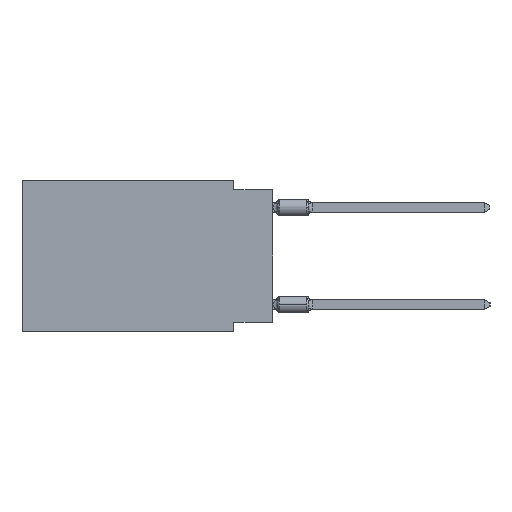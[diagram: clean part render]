
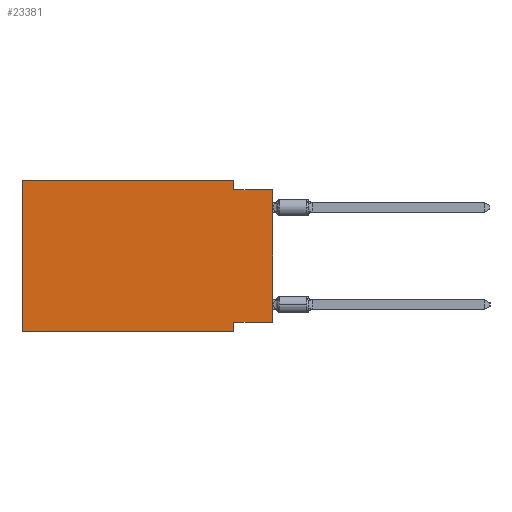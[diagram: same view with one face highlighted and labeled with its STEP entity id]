
A CAD part, left-side view. The second image highlights one B-rep face of the part: STEP entity #23381.
In plain terms, the highlighted planar face has unit normal (-1, 0, 0).
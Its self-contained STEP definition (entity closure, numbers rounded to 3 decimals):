
#74 = LINE ( 'NONE', #25284, #29090 ) ;
#258 = DIRECTION ( 'NONE',  ( 0., 0., 1. ) ) ;
#794 = DIRECTION ( 'NONE',  ( 0., 1., 0. ) ) ;
#1066 = VERTEX_POINT ( 'NONE', #29072 ) ;
#2124 = DIRECTION ( 'NONE',  ( 0., -1., 0. ) ) ;
#2370 = EDGE_CURVE ( 'NONE', #1066, #18489, #74, .T. ) ;
#3048 = LINE ( 'NONE', #8605, #16916 ) ;
#3217 = CARTESIAN_POINT ( 'NONE',  ( 0., 2.54, -0.635 ) ) ;
#3464 = EDGE_CURVE ( 'NONE', #25221, #15336, #23334, .T. ) ;
#4582 = ORIENTED_EDGE ( 'NONE', *, *, #31115, .F. ) ;
#4725 = DIRECTION ( 'NONE',  ( 0., -1., 0. ) ) ;
#5016 = DIRECTION ( 'NONE',  ( 0., 0., -1. ) ) ;
#5195 = DIRECTION ( 'NONE',  ( 1., 0., 0. ) ) ;
#6644 = VECTOR ( 'NONE', #794, 1000. ) ;
#6961 = VECTOR ( 'NONE', #2124, 1000. ) ;
#7699 = PLANE ( 'NONE',  #22214 ) ;
#8605 = CARTESIAN_POINT ( 'NONE',  ( 0., 16.383, 0. ) ) ;
#9693 = LINE ( 'NONE', #28014, #6644 ) ;
#10263 = EDGE_CURVE ( 'NONE', #18567, #1066, #9693, .T. ) ;
#10994 = CARTESIAN_POINT ( 'NONE',  ( 0., 16.383, 0. ) ) ;
#12427 = CARTESIAN_POINT ( 'NONE',  ( 0., 16.383, 0. ) ) ;
#13568 = LINE ( 'NONE', #24493, #6961 ) ;
#13570 = CARTESIAN_POINT ( 'NONE',  ( 0., 0., -0.635 ) ) ;
#14565 = VECTOR ( 'NONE', #5016, 1000. ) ;
#14622 = ORIENTED_EDGE ( 'NONE', *, *, #10263, .F. ) ;
#14913 = DIRECTION ( 'NONE',  ( 0., 0., 1. ) ) ;
#14944 = CARTESIAN_POINT ( 'NONE',  ( 0., 2.54, -9.906 ) ) ;
#14964 = VECTOR ( 'NONE', #4725, 1000. ) ;
#15336 = VERTEX_POINT ( 'NONE', #10994 ) ;
#16800 = DIRECTION ( 'NONE',  ( 0., -1., 0. ) ) ;
#16916 = VECTOR ( 'NONE', #16800, 1000. ) ;
#16941 = CARTESIAN_POINT ( 'NONE',  ( 0., 16.383, -9.906 ) ) ;
#17483 = LINE ( 'NONE', #28431, #14964 ) ;
#17745 = ORIENTED_EDGE ( 'NONE', *, *, #32402, .F. ) ;
#18145 = ORIENTED_EDGE ( 'NONE', *, *, #30326, .T. ) ;
#18489 = VERTEX_POINT ( 'NONE', #14944 ) ;
#18567 = VERTEX_POINT ( 'NONE', #28911 ) ;
#21264 = VERTEX_POINT ( 'NONE', #13570 ) ;
#21716 = ORIENTED_EDGE ( 'NONE', *, *, #25077, .T. ) ;
#22214 = AXIS2_PLACEMENT_3D ( 'NONE', #29540, #5195, #27568 ) ;
#23334 = LINE ( 'NONE', #12427, #29685 ) ;
#23381 = ADVANCED_FACE ( 'NONE', ( #31868 ), #7699, .F. ) ;
#24274 = VECTOR ( 'NONE', #258, 1000. ) ;
#24493 = CARTESIAN_POINT ( 'NONE',  ( 0., 16.383, -9.906 ) ) ;
#24734 = VERTEX_POINT ( 'NONE', #28099 ) ;
#24772 = CARTESIAN_POINT ( 'NONE',  ( 0., 0., 0. ) ) ;
#25077 = EDGE_CURVE ( 'NONE', #25221, #18489, #13568, .T. ) ;
#25221 = VERTEX_POINT ( 'NONE', #16941 ) ;
#25284 = CARTESIAN_POINT ( 'NONE',  ( 0., 2.54, -9.906 ) ) ;
#26261 = ORIENTED_EDGE ( 'NONE', *, *, #3464, .F. ) ;
#26264 = VERTEX_POINT ( 'NONE', #3217 ) ;
#26872 = EDGE_CURVE ( 'NONE', #26264, #21264, #17483, .T. ) ;
#27568 = DIRECTION ( 'NONE',  ( 0., 0., -1. ) ) ;
#27635 = DIRECTION ( 'NONE',  ( 0., 0., -1. ) ) ;
#28014 = CARTESIAN_POINT ( 'NONE',  ( 0., 0., -9.271 ) ) ;
#28099 = CARTESIAN_POINT ( 'NONE',  ( 0., 2.54, 0. ) ) ;
#28231 = ORIENTED_EDGE ( 'NONE', *, *, #2370, .F. ) ;
#28431 = CARTESIAN_POINT ( 'NONE',  ( 0., 0., -0.635 ) ) ;
#28911 = CARTESIAN_POINT ( 'NONE',  ( 0., 0., -9.271 ) ) ;
#29072 = CARTESIAN_POINT ( 'NONE',  ( 0., 2.54, -9.271 ) ) ;
#29090 = VECTOR ( 'NONE', #27635, 1000. ) ;
#29540 = CARTESIAN_POINT ( 'NONE',  ( 0., 16.383, 0. ) ) ;
#29685 = VECTOR ( 'NONE', #14913, 1000. ) ;
#30326 = EDGE_CURVE ( 'NONE', #18567, #21264, #32838, .T. ) ;
#31115 = EDGE_CURVE ( 'NONE', #24734, #26264, #32581, .T. ) ;
#31868 = FACE_OUTER_BOUND ( 'NONE', #34040, .T. ) ;
#32402 = EDGE_CURVE ( 'NONE', #15336, #24734, #3048, .T. ) ;
#32581 = LINE ( 'NONE', #35079, #14565 ) ;
#32838 = LINE ( 'NONE', #24772, #24274 ) ;
#33961 = ORIENTED_EDGE ( 'NONE', *, *, #26872, .F. ) ;
#34040 = EDGE_LOOP ( 'NONE', ( #18145, #33961, #4582, #17745, #26261, #21716, #28231, #14622 ) ) ;
#35079 = CARTESIAN_POINT ( 'NONE',  ( 0., 2.54, 0. ) ) ;
